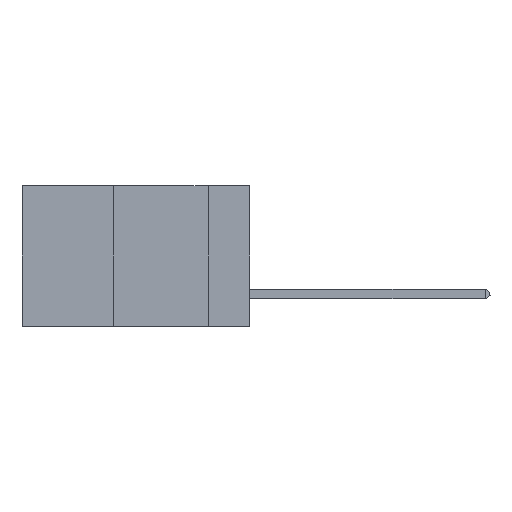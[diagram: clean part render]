
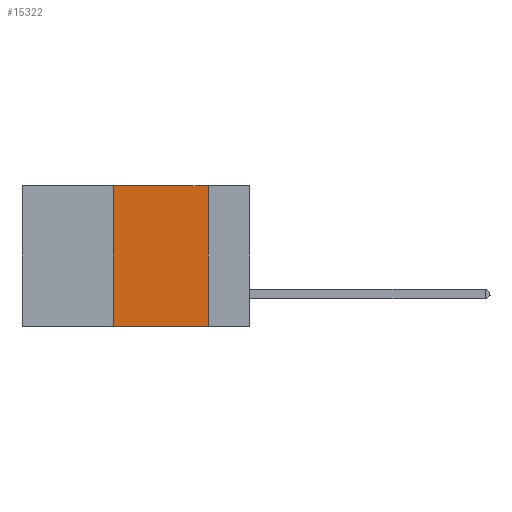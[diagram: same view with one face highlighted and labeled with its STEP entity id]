
A CAD part, left-side view. The second image highlights one B-rep face of the part: STEP entity #15322.
In plain terms, the highlighted planar face has unit normal (-1, 0, 0).
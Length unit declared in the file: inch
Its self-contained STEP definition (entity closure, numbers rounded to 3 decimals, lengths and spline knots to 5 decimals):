
#1533 = FACE_OUTER_BOUND ( 'NONE', #32093, .T. ) ;
#1959 = LINE ( 'NONE', #7089, #24591 ) ;
#4382 = DIRECTION ( 'NONE',  ( 0., 0., -1. ) ) ;
#4950 = ORIENTED_EDGE ( 'NONE', *, *, #18711, .F. ) ;
#6122 = CARTESIAN_POINT ( 'NONE',  ( 0., 0.6, 0. ) ) ;
#7089 = CARTESIAN_POINT ( 'NONE',  ( 0., 0.6, 0. ) ) ;
#8113 = ORIENTED_EDGE ( 'NONE', *, *, #30399, .F. ) ;
#8727 = DIRECTION ( 'NONE',  ( 1., 0., 0. ) ) ;
#9195 = VERTEX_POINT ( 'NONE', #30604 ) ;
#9540 = LINE ( 'NONE', #13412, #30981 ) ;
#10061 = DIRECTION ( 'NONE',  ( 0., 0., 1. ) ) ;
#12085 = CARTESIAN_POINT ( 'NONE',  ( 0., 0.36, -0.37 ) ) ;
#12536 = CARTESIAN_POINT ( 'NONE',  ( 0., 0.11, 0. ) ) ;
#13412 = CARTESIAN_POINT ( 'NONE',  ( 0., 0.6, -0.37 ) ) ;
#13688 = LINE ( 'NONE', #25836, #16121 ) ;
#14416 = VERTEX_POINT ( 'NONE', #15255 ) ;
#15255 = CARTESIAN_POINT ( 'NONE',  ( 0., 0.11, 0. ) ) ;
#15322 = ADVANCED_FACE ( 'NONE', ( #1533 ), #27253, .F. ) ;
#16121 = VECTOR ( 'NONE', #10061, 39.37008 ) ;
#18711 = EDGE_CURVE ( 'NONE', #14416, #9195, #28587, .T. ) ;
#19755 = EDGE_CURVE ( 'NONE', #28232, #9195, #9540, .T. ) ;
#19969 = DIRECTION ( 'NONE',  ( 0., -1., 0. ) ) ;
#20331 = AXIS2_PLACEMENT_3D ( 'NONE', #6122, #8727, #26797 ) ;
#20488 = VECTOR ( 'NONE', #4382, 39.37008 ) ;
#22042 = ORIENTED_EDGE ( 'NONE', *, *, #19755, .T. ) ;
#23023 = CARTESIAN_POINT ( 'NONE',  ( 0., 0.36, 0. ) ) ;
#24191 = ORIENTED_EDGE ( 'NONE', *, *, #29844, .F. ) ;
#24591 = VECTOR ( 'NONE', #33005, 39.37008 ) ;
#25836 = CARTESIAN_POINT ( 'NONE',  ( 0., 0.36, 0. ) ) ;
#26797 = DIRECTION ( 'NONE',  ( 0., 0., -1. ) ) ;
#27253 = PLANE ( 'NONE',  #20331 ) ;
#28232 = VERTEX_POINT ( 'NONE', #12085 ) ;
#28587 = LINE ( 'NONE', #12536, #20488 ) ;
#29786 = VERTEX_POINT ( 'NONE', #23023 ) ;
#29844 = EDGE_CURVE ( 'NONE', #28232, #29786, #13688, .T. ) ;
#30399 = EDGE_CURVE ( 'NONE', #29786, #14416, #1959, .T. ) ;
#30604 = CARTESIAN_POINT ( 'NONE',  ( 0., 0.11, -0.37 ) ) ;
#30981 = VECTOR ( 'NONE', #19969, 39.37008 ) ;
#32093 = EDGE_LOOP ( 'NONE', ( #4950, #8113, #24191, #22042 ) ) ;
#33005 = DIRECTION ( 'NONE',  ( 0., -1., 0. ) ) ;
